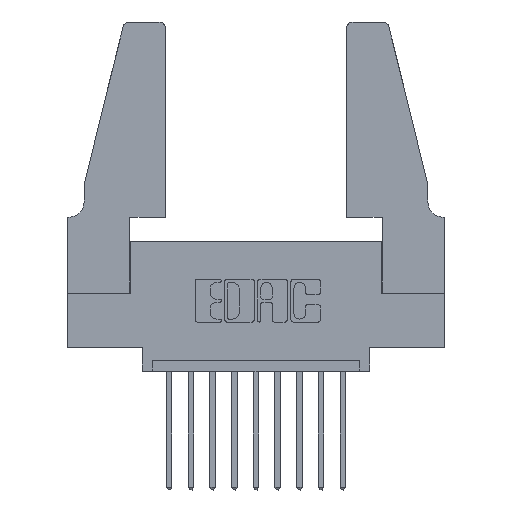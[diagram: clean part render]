
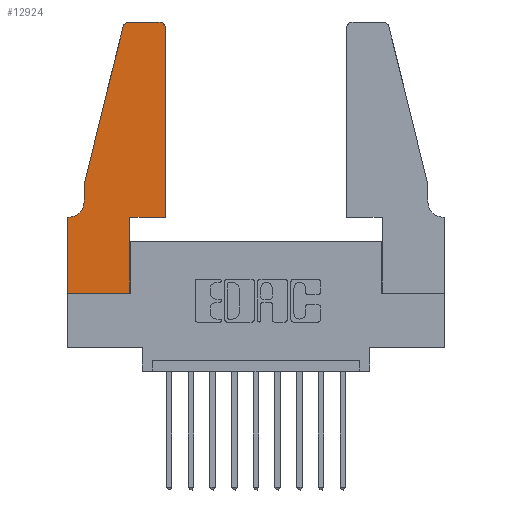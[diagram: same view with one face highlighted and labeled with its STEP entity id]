
A CAD part, top view. The second image highlights one B-rep face of the part: STEP entity #12924.
In plain terms, the highlighted planar face has unit normal (0, 0, 1).
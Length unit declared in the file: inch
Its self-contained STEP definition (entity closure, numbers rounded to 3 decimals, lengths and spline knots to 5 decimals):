
#269 = VECTOR ( 'NONE', #7083, 39.37008 ) ;
#473 = DIRECTION ( 'NONE',  ( 1., 0., 0. ) ) ;
#520 = CARTESIAN_POINT ( 'NONE',  ( 0.2865, 0., 0.37 ) ) ;
#538 = VERTEX_POINT ( 'NONE', #11978 ) ;
#574 = EDGE_LOOP ( 'NONE', ( #931, #1622, #11806, #3266, #9542, #2528, #4113, #3045, #2598, #3161, #5146, #1247 ) ) ;
#764 = EDGE_CURVE ( 'NONE', #12505, #11898, #4792, .T. ) ;
#854 = CIRCLE ( 'NONE', #5880, 0.03 ) ;
#931 = ORIENTED_EDGE ( 'NONE', *, *, #764, .T. ) ;
#965 = LINE ( 'NONE', #10855, #12102 ) ;
#1247 = ORIENTED_EDGE ( 'NONE', *, *, #9662, .T. ) ;
#1622 = ORIENTED_EDGE ( 'NONE', *, *, #8337, .T. ) ;
#1868 = CARTESIAN_POINT ( 'NONE',  ( 0.284, 1.25, 0.37 ) ) ;
#1945 = LINE ( 'NONE', #2361, #9961 ) ;
#1988 = CIRCLE ( 'NONE', #7227, 0.03 ) ;
#2239 = FACE_OUTER_BOUND ( 'NONE', #574, .T. ) ;
#2249 = VERTEX_POINT ( 'NONE', #3227 ) ;
#2361 = CARTESIAN_POINT ( 'NONE',  ( 0., 0., 0.37 ) ) ;
#2528 = ORIENTED_EDGE ( 'NONE', *, *, #12912, .T. ) ;
#2598 = ORIENTED_EDGE ( 'NONE', *, *, #4462, .T. ) ;
#2688 = EDGE_CURVE ( 'NONE', #538, #3245, #4856, .T. ) ;
#2726 = AXIS2_PLACEMENT_3D ( 'NONE', #10851, #4600, #3435 ) ;
#2785 = EDGE_CURVE ( 'NONE', #11256, #10384, #9134, .T. ) ;
#2903 = CARTESIAN_POINT ( 'NONE',  ( 0.4505, 0.35, 0.37 ) ) ;
#3002 = DIRECTION ( 'NONE',  ( 0., 0., -1. ) ) ;
#3045 = ORIENTED_EDGE ( 'NONE', *, *, #10392, .T. ) ;
#3102 = VERTEX_POINT ( 'NONE', #5547 ) ;
#3161 = ORIENTED_EDGE ( 'NONE', *, *, #3819, .T. ) ;
#3227 = CARTESIAN_POINT ( 'NONE',  ( 0., 0.35, 0.37 ) ) ;
#3245 = VERTEX_POINT ( 'NONE', #6059 ) ;
#3266 = ORIENTED_EDGE ( 'NONE', *, *, #10372, .T. ) ;
#3284 = CARTESIAN_POINT ( 'NONE',  ( 0.4505, 0.35, 0.37 ) ) ;
#3435 = DIRECTION ( 'NONE',  ( 1., 0., 0. ) ) ;
#3560 = AXIS2_PLACEMENT_3D ( 'NONE', #13401, #3002, #9192 ) ;
#3657 = DIRECTION ( 'NONE',  ( 0., -1., 0. ) ) ;
#3819 = EDGE_CURVE ( 'NONE', #3102, #11256, #9104, .T. ) ;
#4113 = ORIENTED_EDGE ( 'NONE', *, *, #10959, .T. ) ;
#4215 = CARTESIAN_POINT ( 'NONE',  ( 0.0755, 0.42, 0.37 ) ) ;
#4462 = EDGE_CURVE ( 'NONE', #5342, #3102, #7249, .T. ) ;
#4491 = VERTEX_POINT ( 'NONE', #12016 ) ;
#4600 = DIRECTION ( 'NONE',  ( 0., 0., 1. ) ) ;
#4792 = LINE ( 'NONE', #6216, #12842 ) ;
#4856 = LINE ( 'NONE', #10302, #5481 ) ;
#4888 = CARTESIAN_POINT ( 'NONE',  ( 0.4505, 0.35, 0.37 ) ) ;
#5146 = ORIENTED_EDGE ( 'NONE', *, *, #2785, .T. ) ;
#5305 = DIRECTION ( 'NONE',  ( 0., 1., 0. ) ) ;
#5342 = VERTEX_POINT ( 'NONE', #520 ) ;
#5423 = VECTOR ( 'NONE', #13165, 39.37008 ) ;
#5481 = VECTOR ( 'NONE', #6099, 39.37008 ) ;
#5547 = CARTESIAN_POINT ( 'NONE',  ( 0.2865, 0.35, 0.37 ) ) ;
#5859 = DIRECTION ( 'NONE',  ( 0., 0., 1. ) ) ;
#5880 = AXIS2_PLACEMENT_3D ( 'NONE', #9980, #5859, #473 ) ;
#6059 = CARTESIAN_POINT ( 'NONE',  ( 0.0755, 0.5, 0.37 ) ) ;
#6099 = DIRECTION ( 'NONE',  ( -0.239, -0.971, 0. ) ) ;
#6216 = CARTESIAN_POINT ( 'NONE',  ( 0.2605, 1.25, 0.37 ) ) ;
#6322 = LINE ( 'NONE', #7773, #7175 ) ;
#6938 = VERTEX_POINT ( 'NONE', #8398 ) ;
#7083 = DIRECTION ( 'NONE',  ( 1., 0., 0. ) ) ;
#7175 = VECTOR ( 'NONE', #11911, 39.37008 ) ;
#7227 = AXIS2_PLACEMENT_3D ( 'NONE', #13030, #10921, #12982 ) ;
#7249 = LINE ( 'NONE', #10014, #5423 ) ;
#7428 = VERTEX_POINT ( 'NONE', #4215 ) ;
#7773 = CARTESIAN_POINT ( 'NONE',  ( 0., 0., 0.37 ) ) ;
#8337 = EDGE_CURVE ( 'NONE', #11898, #538, #854, .T. ) ;
#8398 = CARTESIAN_POINT ( 'NONE',  ( 0., 0., 0.37 ) ) ;
#8642 = CIRCLE ( 'NONE', #3560, 0.07 ) ;
#8656 = PLANE ( 'NONE',  #2726 ) ;
#9104 = LINE ( 'NONE', #2903, #269 ) ;
#9134 = LINE ( 'NONE', #3284, #10436 ) ;
#9192 = DIRECTION ( 'NONE',  ( -1., 0., 0. ) ) ;
#9325 = DIRECTION ( 'NONE',  ( -1., 0., 0. ) ) ;
#9542 = ORIENTED_EDGE ( 'NONE', *, *, #10815, .T. ) ;
#9662 = EDGE_CURVE ( 'NONE', #10384, #12505, #1988, .T. ) ;
#9961 = VECTOR ( 'NONE', #12836, 39.37008 ) ;
#9980 = CARTESIAN_POINT ( 'NONE',  ( 0.284, 1.22, 0.37 ) ) ;
#10014 = CARTESIAN_POINT ( 'NONE',  ( 0.2865, 0.35, 0.37 ) ) ;
#10078 = LINE ( 'NONE', #12966, #10908 ) ;
#10302 = CARTESIAN_POINT ( 'NONE',  ( 0.0755, 0.5, 0.37 ) ) ;
#10372 = EDGE_CURVE ( 'NONE', #3245, #7428, #965, .T. ) ;
#10384 = VERTEX_POINT ( 'NONE', #11957 ) ;
#10392 = EDGE_CURVE ( 'NONE', #6938, #5342, #6322, .T. ) ;
#10436 = VECTOR ( 'NONE', #5305, 39.37008 ) ;
#10815 = EDGE_CURVE ( 'NONE', #7428, #4491, #8642, .T. ) ;
#10851 = CARTESIAN_POINT ( 'NONE',  ( 0., 0.35, 0.37 ) ) ;
#10855 = CARTESIAN_POINT ( 'NONE',  ( 0.0755, 0.5, 0.37 ) ) ;
#10900 = DIRECTION ( 'NONE',  ( -1., 0., 0. ) ) ;
#10908 = VECTOR ( 'NONE', #10900, 39.37008 ) ;
#10921 = DIRECTION ( 'NONE',  ( 0., 0., 1. ) ) ;
#10959 = EDGE_CURVE ( 'NONE', #2249, #6938, #1945, .T. ) ;
#11256 = VERTEX_POINT ( 'NONE', #4888 ) ;
#11806 = ORIENTED_EDGE ( 'NONE', *, *, #2688, .T. ) ;
#11898 = VERTEX_POINT ( 'NONE', #1868 ) ;
#11911 = DIRECTION ( 'NONE',  ( 1., 0., 0. ) ) ;
#11957 = CARTESIAN_POINT ( 'NONE',  ( 0.4505, 1.22, 0.37 ) ) ;
#11978 = CARTESIAN_POINT ( 'NONE',  ( 0.25487, 1.22718, 0.37 ) ) ;
#12016 = CARTESIAN_POINT ( 'NONE',  ( 0.0055, 0.35, 0.37 ) ) ;
#12102 = VECTOR ( 'NONE', #3657, 39.37008 ) ;
#12292 = CARTESIAN_POINT ( 'NONE',  ( 0.4205, 1.25, 0.37 ) ) ;
#12505 = VERTEX_POINT ( 'NONE', #12292 ) ;
#12836 = DIRECTION ( 'NONE',  ( 0., -1., 0. ) ) ;
#12842 = VECTOR ( 'NONE', #9325, 39.37008 ) ;
#12912 = EDGE_CURVE ( 'NONE', #4491, #2249, #10078, .T. ) ;
#12924 = ADVANCED_FACE ( 'NONE', ( #2239 ), #8656, .T. ) ;
#12966 = CARTESIAN_POINT ( 'NONE',  ( 0.0755, 0.35, 0.37 ) ) ;
#12982 = DIRECTION ( 'NONE',  ( 1., 0., 0. ) ) ;
#13030 = CARTESIAN_POINT ( 'NONE',  ( 0.4205, 1.22, 0.37 ) ) ;
#13165 = DIRECTION ( 'NONE',  ( 0., 1., 0. ) ) ;
#13401 = CARTESIAN_POINT ( 'NONE',  ( 0.0055, 0.42, 0.37 ) ) ;
